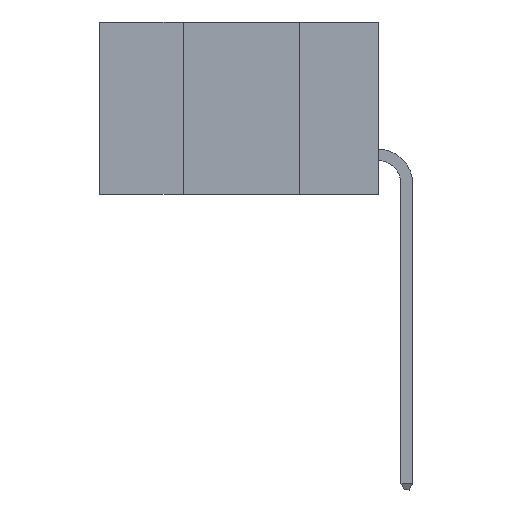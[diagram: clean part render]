
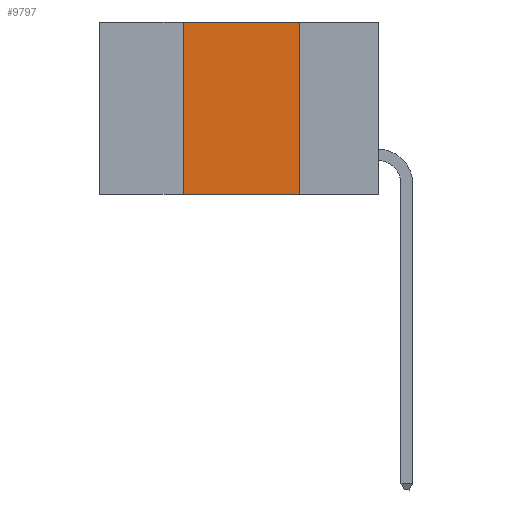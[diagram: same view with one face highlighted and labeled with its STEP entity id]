
A CAD part, left-side view. The second image highlights one B-rep face of the part: STEP entity #9797.
In plain terms, the highlighted planar face has unit normal (-1, 0, 0).
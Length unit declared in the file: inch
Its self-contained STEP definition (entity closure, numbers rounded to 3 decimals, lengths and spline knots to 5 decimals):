
#100 = EDGE_CURVE ( 'NONE', #715, #14468, #8605, .T. ) ;
#623 = DIRECTION ( 'NONE',  ( 0., 0., -1. ) ) ;
#643 = AXIS2_PLACEMENT_3D ( 'NONE', #6826, #7962, #623 ) ;
#715 = VERTEX_POINT ( 'NONE', #9873 ) ;
#1974 = CARTESIAN_POINT ( 'NONE',  ( 0., 0.6, 0. ) ) ;
#2063 = CARTESIAN_POINT ( 'NONE',  ( 0., 0.17, 0. ) ) ;
#2253 = VERTEX_POINT ( 'NONE', #9657 ) ;
#2864 = LINE ( 'NONE', #7615, #14443 ) ;
#3210 = CARTESIAN_POINT ( 'NONE',  ( 0., 0.42, 0. ) ) ;
#3360 = DIRECTION ( 'NONE',  ( 0., -1., 0. ) ) ;
#3374 = ORIENTED_EDGE ( 'NONE', *, *, #8311, .F. ) ;
#3433 = DIRECTION ( 'NONE',  ( 0., 0., -1. ) ) ;
#3607 = ORIENTED_EDGE ( 'NONE', *, *, #13031, .F. ) ;
#4088 = DIRECTION ( 'NONE',  ( 0., 0., 1. ) ) ;
#5708 = FACE_OUTER_BOUND ( 'NONE', #9526, .T. ) ;
#6826 = CARTESIAN_POINT ( 'NONE',  ( 0., 0.6, 0. ) ) ;
#6851 = LINE ( 'NONE', #2063, #9426 ) ;
#7081 = VERTEX_POINT ( 'NONE', #3210 ) ;
#7555 = ORIENTED_EDGE ( 'NONE', *, *, #100, .T. ) ;
#7615 = CARTESIAN_POINT ( 'NONE',  ( 0., 0.42, 0. ) ) ;
#7962 = DIRECTION ( 'NONE',  ( 1., 0., 0. ) ) ;
#8275 = VECTOR ( 'NONE', #3360, 39.37008 ) ;
#8311 = EDGE_CURVE ( 'NONE', #7081, #2253, #12071, .T. ) ;
#8427 = ORIENTED_EDGE ( 'NONE', *, *, #11865, .F. ) ;
#8605 = LINE ( 'NONE', #9535, #8275 ) ;
#9114 = DIRECTION ( 'NONE',  ( 0., -1., 0. ) ) ;
#9426 = VECTOR ( 'NONE', #3433, 39.37008 ) ;
#9526 = EDGE_LOOP ( 'NONE', ( #3607, #3374, #8427, #7555 ) ) ;
#9535 = CARTESIAN_POINT ( 'NONE',  ( 0., 0.6, -0.37 ) ) ;
#9657 = CARTESIAN_POINT ( 'NONE',  ( 0., 0.17, 0. ) ) ;
#9797 = ADVANCED_FACE ( 'NONE', ( #5708 ), #13301, .F. ) ;
#9873 = CARTESIAN_POINT ( 'NONE',  ( 0., 0.42, -0.37 ) ) ;
#10035 = CARTESIAN_POINT ( 'NONE',  ( 0., 0.17, -0.37 ) ) ;
#11865 = EDGE_CURVE ( 'NONE', #715, #7081, #2864, .T. ) ;
#12071 = LINE ( 'NONE', #1974, #14543 ) ;
#13031 = EDGE_CURVE ( 'NONE', #2253, #14468, #6851, .T. ) ;
#13301 = PLANE ( 'NONE',  #643 ) ;
#14443 = VECTOR ( 'NONE', #4088, 39.37008 ) ;
#14468 = VERTEX_POINT ( 'NONE', #10035 ) ;
#14543 = VECTOR ( 'NONE', #9114, 39.37008 ) ;
